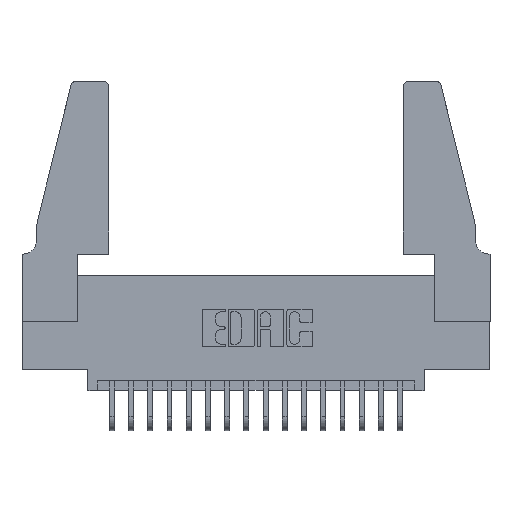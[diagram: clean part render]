
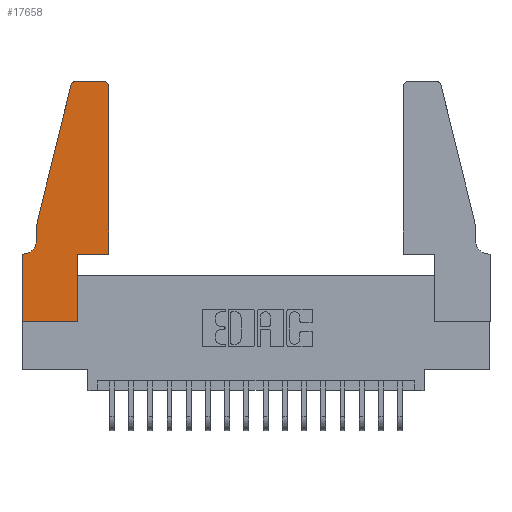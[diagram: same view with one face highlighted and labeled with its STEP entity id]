
A CAD part, top view. The second image highlights one B-rep face of the part: STEP entity #17658.
In plain terms, the highlighted planar face has unit normal (0, 0, 1).
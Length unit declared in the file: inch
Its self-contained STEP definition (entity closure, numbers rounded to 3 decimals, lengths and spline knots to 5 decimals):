
#116 = DIRECTION ( 'NONE',  ( 0., 0., -1. ) ) ;
#252 = CIRCLE ( 'NONE', #14480, 0.03 ) ;
#420 = ORIENTED_EDGE ( 'NONE', *, *, #15928, .T. ) ;
#638 = CARTESIAN_POINT ( 'NONE',  ( 0.4505, 1.22, 0.37 ) ) ;
#735 = CARTESIAN_POINT ( 'NONE',  ( 0.0055, 0.35, 0.37 ) ) ;
#1152 = DIRECTION ( 'NONE',  ( 0., 0., 1. ) ) ;
#1188 = EDGE_CURVE ( 'NONE', #14754, #1997, #11268, .T. ) ;
#1289 = VECTOR ( 'NONE', #13438, 39.37008 ) ;
#1352 = DIRECTION ( 'NONE',  ( -1., 0., 0. ) ) ;
#1608 = DIRECTION ( 'NONE',  ( -1., 0., 0. ) ) ;
#1611 = ORIENTED_EDGE ( 'NONE', *, *, #2765, .T. ) ;
#1913 = ORIENTED_EDGE ( 'NONE', *, *, #1188, .T. ) ;
#1937 = VERTEX_POINT ( 'NONE', #638 ) ;
#1997 = VERTEX_POINT ( 'NONE', #10316 ) ;
#2178 = CARTESIAN_POINT ( 'NONE',  ( 0.2865, 0.35, 0.37 ) ) ;
#2388 = CARTESIAN_POINT ( 'NONE',  ( 0.2605, 1.25, 0.37 ) ) ;
#2521 = DIRECTION ( 'NONE',  ( 0., 0., 1. ) ) ;
#2765 = EDGE_CURVE ( 'NONE', #17566, #14500, #10762, .T. ) ;
#3003 = CARTESIAN_POINT ( 'NONE',  ( 0.4505, 0.35, 0.37 ) ) ;
#3661 = VECTOR ( 'NONE', #17721, 39.37008 ) ;
#4330 = CIRCLE ( 'NONE', #17359, 0.07 ) ;
#4375 = CARTESIAN_POINT ( 'NONE',  ( 0.4505, 0.35, 0.37 ) ) ;
#4489 = DIRECTION ( 'NONE',  ( 1., 0., 0. ) ) ;
#4490 = VECTOR ( 'NONE', #1352, 39.37008 ) ;
#4657 = LINE ( 'NONE', #4375, #8998 ) ;
#4886 = ORIENTED_EDGE ( 'NONE', *, *, #14013, .T. ) ;
#5215 = LINE ( 'NONE', #7314, #8852 ) ;
#5326 = EDGE_CURVE ( 'NONE', #7981, #14754, #9461, .T. ) ;
#5700 = VERTEX_POINT ( 'NONE', #17671 ) ;
#5702 = FACE_OUTER_BOUND ( 'NONE', #6747, .T. ) ;
#5730 = CARTESIAN_POINT ( 'NONE',  ( 0., 0.35, 0.37 ) ) ;
#5797 = VERTEX_POINT ( 'NONE', #13985 ) ;
#5941 = DIRECTION ( 'NONE',  ( 1., 0., 0. ) ) ;
#6251 = CARTESIAN_POINT ( 'NONE',  ( 0.2865, 0., 0.37 ) ) ;
#6294 = ORIENTED_EDGE ( 'NONE', *, *, #14579, .T. ) ;
#6455 = EDGE_CURVE ( 'NONE', #9889, #11743, #17012, .T. ) ;
#6707 = EDGE_CURVE ( 'NONE', #14500, #5797, #9966, .T. ) ;
#6747 = EDGE_LOOP ( 'NONE', ( #13842, #1913, #14248, #14554, #420, #1611, #13614, #10565, #11090, #6294, #11843, #4886 ) ) ;
#6994 = VERTEX_POINT ( 'NONE', #14639 ) ;
#7314 = CARTESIAN_POINT ( 'NONE',  ( 0.0755, 0.5, 0.37 ) ) ;
#7364 = DIRECTION ( 'NONE',  ( 0., 0., 1. ) ) ;
#7981 = VERTEX_POINT ( 'NONE', #11770 ) ;
#8161 = DIRECTION ( 'NONE',  ( 0., -1., 0. ) ) ;
#8644 = CARTESIAN_POINT ( 'NONE',  ( 0., 0., 0.37 ) ) ;
#8852 = VECTOR ( 'NONE', #16652, 39.37008 ) ;
#8962 = VECTOR ( 'NONE', #8161, 39.37008 ) ;
#8998 = VECTOR ( 'NONE', #5941, 39.37008 ) ;
#9006 = CARTESIAN_POINT ( 'NONE',  ( 0.4205, 1.22, 0.37 ) ) ;
#9461 = LINE ( 'NONE', #2388, #3661 ) ;
#9889 = VERTEX_POINT ( 'NONE', #6251 ) ;
#9891 = LINE ( 'NONE', #14313, #8962 ) ;
#9966 = LINE ( 'NONE', #8644, #16772 ) ;
#10260 = AXIS2_PLACEMENT_3D ( 'NONE', #11735, #2521, #12012 ) ;
#10316 = CARTESIAN_POINT ( 'NONE',  ( 0.25487, 1.22718, 0.37 ) ) ;
#10565 = ORIENTED_EDGE ( 'NONE', *, *, #13363, .T. ) ;
#10762 = LINE ( 'NONE', #13930, #4490 ) ;
#11090 = ORIENTED_EDGE ( 'NONE', *, *, #6455, .T. ) ;
#11268 = CIRCLE ( 'NONE', #11331, 0.03 ) ;
#11331 = AXIS2_PLACEMENT_3D ( 'NONE', #16642, #7364, #18184 ) ;
#11335 = VECTOR ( 'NONE', #12373, 39.37008 ) ;
#11721 = CARTESIAN_POINT ( 'NONE',  ( 0.2865, 0.35, 0.37 ) ) ;
#11735 = CARTESIAN_POINT ( 'NONE',  ( 0., 0.35, 0.37 ) ) ;
#11743 = VERTEX_POINT ( 'NONE', #2178 ) ;
#11770 = CARTESIAN_POINT ( 'NONE',  ( 0.4205, 1.25, 0.37 ) ) ;
#11843 = ORIENTED_EDGE ( 'NONE', *, *, #15356, .T. ) ;
#12012 = DIRECTION ( 'NONE',  ( 1., 0., 0. ) ) ;
#12373 = DIRECTION ( 'NONE',  ( 0., 1., 0. ) ) ;
#12384 = VECTOR ( 'NONE', #4489, 39.37008 ) ;
#12516 = CARTESIAN_POINT ( 'NONE',  ( 0.284, 1.25, 0.37 ) ) ;
#13363 = EDGE_CURVE ( 'NONE', #5797, #9889, #14784, .T. ) ;
#13438 = DIRECTION ( 'NONE',  ( 0., 1., 0. ) ) ;
#13614 = ORIENTED_EDGE ( 'NONE', *, *, #6707, .T. ) ;
#13842 = ORIENTED_EDGE ( 'NONE', *, *, #5326, .T. ) ;
#13930 = CARTESIAN_POINT ( 'NONE',  ( 0.0755, 0.35, 0.37 ) ) ;
#13985 = CARTESIAN_POINT ( 'NONE',  ( 0., 0., 0.37 ) ) ;
#14013 = EDGE_CURVE ( 'NONE', #1937, #7981, #252, .T. ) ;
#14248 = ORIENTED_EDGE ( 'NONE', *, *, #17829, .T. ) ;
#14313 = CARTESIAN_POINT ( 'NONE',  ( 0.0755, 0.5, 0.37 ) ) ;
#14480 = AXIS2_PLACEMENT_3D ( 'NONE', #9006, #1152, #14976 ) ;
#14500 = VERTEX_POINT ( 'NONE', #5730 ) ;
#14554 = ORIENTED_EDGE ( 'NONE', *, *, #15682, .T. ) ;
#14579 = EDGE_CURVE ( 'NONE', #11743, #16651, #4657, .T. ) ;
#14639 = CARTESIAN_POINT ( 'NONE',  ( 0.0755, 0.5, 0.37 ) ) ;
#14754 = VERTEX_POINT ( 'NONE', #12516 ) ;
#14784 = LINE ( 'NONE', #18353, #12384 ) ;
#14976 = DIRECTION ( 'NONE',  ( 1., 0., 0. ) ) ;
#15356 = EDGE_CURVE ( 'NONE', #16651, #1937, #18398, .T. ) ;
#15682 = EDGE_CURVE ( 'NONE', #6994, #5700, #9891, .T. ) ;
#15928 = EDGE_CURVE ( 'NONE', #5700, #17566, #4330, .T. ) ;
#16642 = CARTESIAN_POINT ( 'NONE',  ( 0.284, 1.22, 0.37 ) ) ;
#16651 = VERTEX_POINT ( 'NONE', #17190 ) ;
#16652 = DIRECTION ( 'NONE',  ( -0.239, -0.971, 0. ) ) ;
#16772 = VECTOR ( 'NONE', #19526, 39.37008 ) ;
#16892 = CARTESIAN_POINT ( 'NONE',  ( 0.0055, 0.42, 0.37 ) ) ;
#17012 = LINE ( 'NONE', #11721, #1289 ) ;
#17190 = CARTESIAN_POINT ( 'NONE',  ( 0.4505, 0.35, 0.37 ) ) ;
#17359 = AXIS2_PLACEMENT_3D ( 'NONE', #16892, #116, #1608 ) ;
#17566 = VERTEX_POINT ( 'NONE', #735 ) ;
#17658 = ADVANCED_FACE ( 'NONE', ( #5702 ), #18187, .T. ) ;
#17671 = CARTESIAN_POINT ( 'NONE',  ( 0.0755, 0.42, 0.37 ) ) ;
#17721 = DIRECTION ( 'NONE',  ( -1., 0., 0. ) ) ;
#17829 = EDGE_CURVE ( 'NONE', #1997, #6994, #5215, .T. ) ;
#18184 = DIRECTION ( 'NONE',  ( 1., 0., 0. ) ) ;
#18187 = PLANE ( 'NONE',  #10260 ) ;
#18353 = CARTESIAN_POINT ( 'NONE',  ( 0., 0., 0.37 ) ) ;
#18398 = LINE ( 'NONE', #3003, #11335 ) ;
#19526 = DIRECTION ( 'NONE',  ( 0., -1., 0. ) ) ;
